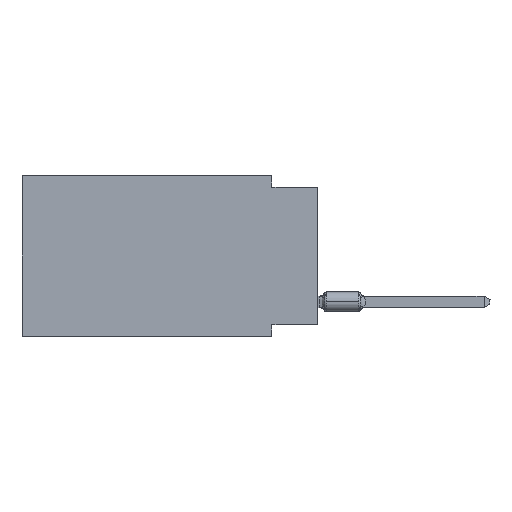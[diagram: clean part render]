
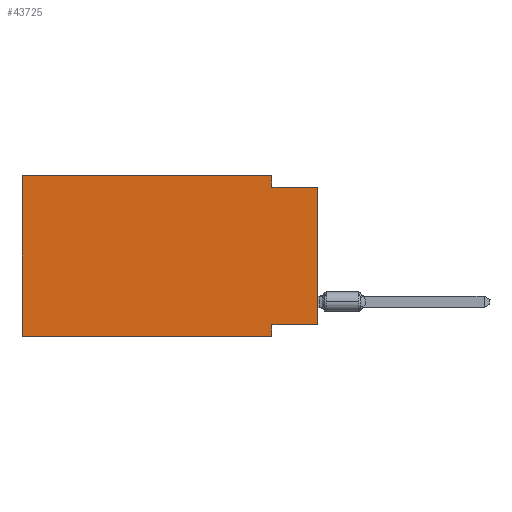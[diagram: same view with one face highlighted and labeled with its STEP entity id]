
A CAD part, left-side view. The second image highlights one B-rep face of the part: STEP entity #43725.
In plain terms, the highlighted planar face has unit normal (-1, 0, 0).
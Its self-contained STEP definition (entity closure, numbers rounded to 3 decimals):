
#688 = ORIENTED_EDGE ( 'NONE', *, *, #23941, .F. ) ;
#860 = DIRECTION ( 'NONE',  ( 0., -1., 0. ) ) ;
#900 = ORIENTED_EDGE ( 'NONE', *, *, #44608, .F. ) ;
#1346 = LINE ( 'NONE', #45686, #23102 ) ;
#1542 = VECTOR ( 'NONE', #45383, 1000. ) ;
#2053 = DIRECTION ( 'NONE',  ( 0., 0., 1. ) ) ;
#3124 = EDGE_LOOP ( 'NONE', ( #3392, #36033, #18665, #688, #24753, #17020, #9109, #900 ) ) ;
#3392 = ORIENTED_EDGE ( 'NONE', *, *, #22238, .T. ) ;
#4330 = VERTEX_POINT ( 'NONE', #43798 ) ;
#6242 = LINE ( 'NONE', #42789, #14044 ) ;
#8417 = DIRECTION ( 'NONE',  ( 0., 0., -1. ) ) ;
#9109 = ORIENTED_EDGE ( 'NONE', *, *, #42155, .F. ) ;
#12041 = CARTESIAN_POINT ( 'NONE',  ( 0., 16.383, 0. ) ) ;
#12102 = DIRECTION ( 'NONE',  ( 0., 1., 0. ) ) ;
#12541 = LINE ( 'NONE', #35440, #44394 ) ;
#12912 = CARTESIAN_POINT ( 'NONE',  ( 0., 2.54, 0. ) ) ;
#14044 = VECTOR ( 'NONE', #28425, 1000. ) ;
#14467 = VERTEX_POINT ( 'NONE', #17633 ) ;
#14610 = LINE ( 'NONE', #34507, #22555 ) ;
#17020 = ORIENTED_EDGE ( 'NONE', *, *, #21444, .T. ) ;
#17633 = CARTESIAN_POINT ( 'NONE',  ( 0., 2.54, 0. ) ) ;
#18378 = PLANE ( 'NONE',  #29869 ) ;
#18665 = ORIENTED_EDGE ( 'NONE', *, *, #36845, .F. ) ;
#20678 = VECTOR ( 'NONE', #43126, 1000. ) ;
#20907 = EDGE_CURVE ( 'NONE', #30569, #4330, #30089, .T. ) ;
#21444 = EDGE_CURVE ( 'NONE', #39054, #27074, #33694, .T. ) ;
#22238 = EDGE_CURVE ( 'NONE', #35720, #4330, #12541, .T. ) ;
#22555 = VECTOR ( 'NONE', #12102, 1000. ) ;
#23102 = VECTOR ( 'NONE', #8417, 1000. ) ;
#23253 = CARTESIAN_POINT ( 'NONE',  ( 0., 0., -0.635 ) ) ;
#23256 = CARTESIAN_POINT ( 'NONE',  ( 0., 16.383, 0. ) ) ;
#23941 = EDGE_CURVE ( 'NONE', #37673, #14467, #6242, .T. ) ;
#24753 = ORIENTED_EDGE ( 'NONE', *, *, #29870, .F. ) ;
#27074 = VERTEX_POINT ( 'NONE', #44701 ) ;
#28425 = DIRECTION ( 'NONE',  ( 0., -1., 0. ) ) ;
#29592 = DIRECTION ( 'NONE',  ( 0., 0., -1. ) ) ;
#29869 = AXIS2_PLACEMENT_3D ( 'NONE', #12041, #37859, #29592 ) ;
#29870 = EDGE_CURVE ( 'NONE', #39054, #37673, #38665, .T. ) ;
#30089 = LINE ( 'NONE', #23253, #35707 ) ;
#30569 = VERTEX_POINT ( 'NONE', #33162 ) ;
#31353 = CARTESIAN_POINT ( 'NONE',  ( 0., 16.383, 0. ) ) ;
#33162 = CARTESIAN_POINT ( 'NONE',  ( 0., 2.54, -0.635 ) ) ;
#33694 = LINE ( 'NONE', #37351, #1542 ) ;
#34507 = CARTESIAN_POINT ( 'NONE',  ( 0., 0., -8.255 ) ) ;
#35440 = CARTESIAN_POINT ( 'NONE',  ( 0., 0., 0. ) ) ;
#35707 = VECTOR ( 'NONE', #860, 1000. ) ;
#35720 = VERTEX_POINT ( 'NONE', #46263 ) ;
#35793 = VERTEX_POINT ( 'NONE', #40648 ) ;
#36033 = ORIENTED_EDGE ( 'NONE', *, *, #20907, .F. ) ;
#36845 = EDGE_CURVE ( 'NONE', #14467, #30569, #39941, .T. ) ;
#37351 = CARTESIAN_POINT ( 'NONE',  ( 0., 16.383, -8.89 ) ) ;
#37370 = VECTOR ( 'NONE', #37938, 1000. ) ;
#37673 = VERTEX_POINT ( 'NONE', #23256 ) ;
#37859 = DIRECTION ( 'NONE',  ( 1., 0., 0. ) ) ;
#37938 = DIRECTION ( 'NONE',  ( 0., 0., 1. ) ) ;
#38665 = LINE ( 'NONE', #31353, #37370 ) ;
#39054 = VERTEX_POINT ( 'NONE', #45835 ) ;
#39941 = LINE ( 'NONE', #12912, #20678 ) ;
#40648 = CARTESIAN_POINT ( 'NONE',  ( 0., 2.54, -8.255 ) ) ;
#42155 = EDGE_CURVE ( 'NONE', #35793, #27074, #1346, .T. ) ;
#42789 = CARTESIAN_POINT ( 'NONE',  ( 0., 16.383, 0. ) ) ;
#43126 = DIRECTION ( 'NONE',  ( 0., 0., -1. ) ) ;
#43725 = ADVANCED_FACE ( 'NONE', ( #45409 ), #18378, .F. ) ;
#43798 = CARTESIAN_POINT ( 'NONE',  ( 0., 0., -0.635 ) ) ;
#44394 = VECTOR ( 'NONE', #2053, 1000. ) ;
#44608 = EDGE_CURVE ( 'NONE', #35720, #35793, #14610, .T. ) ;
#44701 = CARTESIAN_POINT ( 'NONE',  ( 0., 2.54, -8.89 ) ) ;
#45383 = DIRECTION ( 'NONE',  ( 0., -1., 0. ) ) ;
#45409 = FACE_OUTER_BOUND ( 'NONE', #3124, .T. ) ;
#45686 = CARTESIAN_POINT ( 'NONE',  ( 0., 2.54, -8.89 ) ) ;
#45835 = CARTESIAN_POINT ( 'NONE',  ( 0., 16.383, -8.89 ) ) ;
#46263 = CARTESIAN_POINT ( 'NONE',  ( 0., 0., -8.255 ) ) ;
